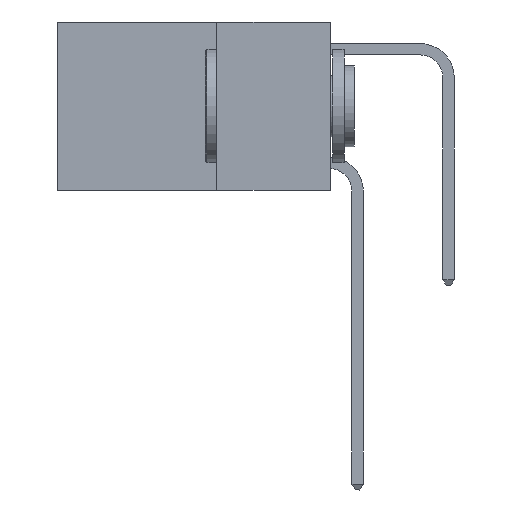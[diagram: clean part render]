
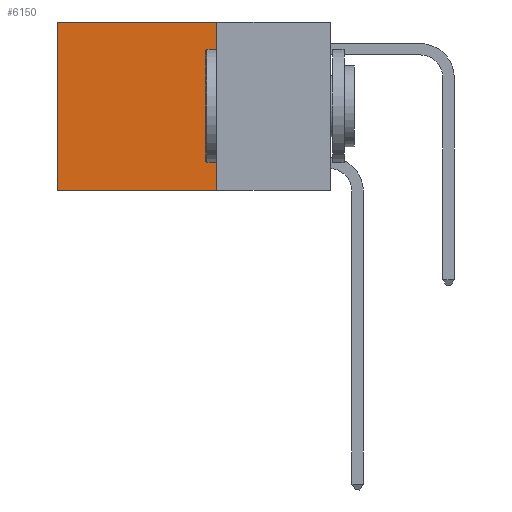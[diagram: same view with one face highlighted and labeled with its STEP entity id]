
A CAD part, left-side view. The second image highlights one B-rep face of the part: STEP entity #6150.
In plain terms, the highlighted planar face has unit normal (-1, 0, 0).
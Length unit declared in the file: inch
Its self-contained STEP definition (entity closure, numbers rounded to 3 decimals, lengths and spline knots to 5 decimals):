
#323 = VECTOR ( 'NONE', #1465, 39.37008 ) ;
#514 = EDGE_CURVE ( 'NONE', #7337, #6662, #4390, .T. ) ;
#672 = LINE ( 'NONE', #10448, #9699 ) ;
#785 = CARTESIAN_POINT ( 'NONE',  ( 0.2625, 0.25, 0. ) ) ;
#1465 = DIRECTION ( 'NONE',  ( 0., 1., 0. ) ) ;
#1617 = CARTESIAN_POINT ( 'NONE',  ( 0.2625, 0.6, -0.37 ) ) ;
#2137 = DIRECTION ( 'NONE',  ( 0., 0., -1. ) ) ;
#3213 = CARTESIAN_POINT ( 'NONE',  ( 0.2625, 0.25, -0.37 ) ) ;
#4130 = EDGE_CURVE ( 'NONE', #14378, #6662, #672, .T. ) ;
#4370 = DIRECTION ( 'NONE',  ( 0., 0., -1. ) ) ;
#4390 = LINE ( 'NONE', #3213, #5195 ) ;
#4483 = VECTOR ( 'NONE', #2137, 39.37008 ) ;
#4524 = CARTESIAN_POINT ( 'NONE',  ( 0.2625, 0.6, 0. ) ) ;
#4600 = DIRECTION ( 'NONE',  ( 1., 0., 0. ) ) ;
#4737 = CARTESIAN_POINT ( 'NONE',  ( 0.2625, 0.25, 0. ) ) ;
#4861 = CARTESIAN_POINT ( 'NONE',  ( 0.2625, 0.25, -0.37 ) ) ;
#5195 = VECTOR ( 'NONE', #8109, 39.37008 ) ;
#5715 = ORIENTED_EDGE ( 'NONE', *, *, #514, .F. ) ;
#6150 = ADVANCED_FACE ( 'NONE', ( #10724 ), #9444, .F. ) ;
#6662 = VERTEX_POINT ( 'NONE', #1617 ) ;
#7337 = VERTEX_POINT ( 'NONE', #4861 ) ;
#7466 = CARTESIAN_POINT ( 'NONE',  ( 0.2625, 0.25, 0. ) ) ;
#8109 = DIRECTION ( 'NONE',  ( 0., 1., 0. ) ) ;
#8278 = VERTEX_POINT ( 'NONE', #4737 ) ;
#9144 = ORIENTED_EDGE ( 'NONE', *, *, #14278, .F. ) ;
#9444 = PLANE ( 'NONE',  #12534 ) ;
#9699 = VECTOR ( 'NONE', #12781, 39.37008 ) ;
#10448 = CARTESIAN_POINT ( 'NONE',  ( 0.2625, 0.6, 0. ) ) ;
#10724 = FACE_OUTER_BOUND ( 'NONE', #13886, .T. ) ;
#10804 = LINE ( 'NONE', #785, #4483 ) ;
#11465 = EDGE_CURVE ( 'NONE', #8278, #14378, #12196, .T. ) ;
#12164 = ORIENTED_EDGE ( 'NONE', *, *, #11465, .T. ) ;
#12196 = LINE ( 'NONE', #7466, #323 ) ;
#12534 = AXIS2_PLACEMENT_3D ( 'NONE', #14293, #4600, #4370 ) ;
#12781 = DIRECTION ( 'NONE',  ( 0., 0., -1. ) ) ;
#13886 = EDGE_LOOP ( 'NONE', ( #15341, #5715, #9144, #12164 ) ) ;
#14278 = EDGE_CURVE ( 'NONE', #8278, #7337, #10804, .T. ) ;
#14293 = CARTESIAN_POINT ( 'NONE',  ( 0.2625, 0.25, 0. ) ) ;
#14378 = VERTEX_POINT ( 'NONE', #4524 ) ;
#15341 = ORIENTED_EDGE ( 'NONE', *, *, #4130, .T. ) ;
